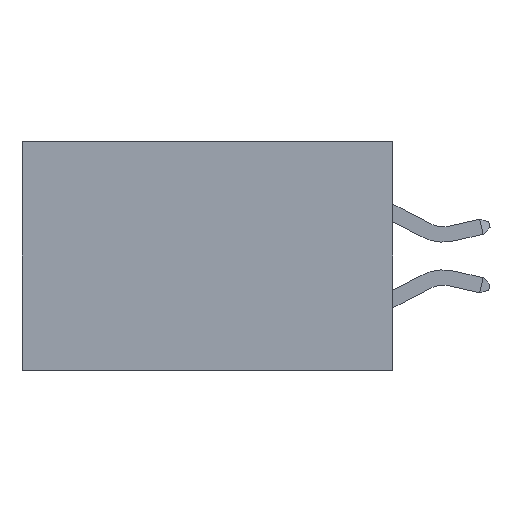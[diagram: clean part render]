
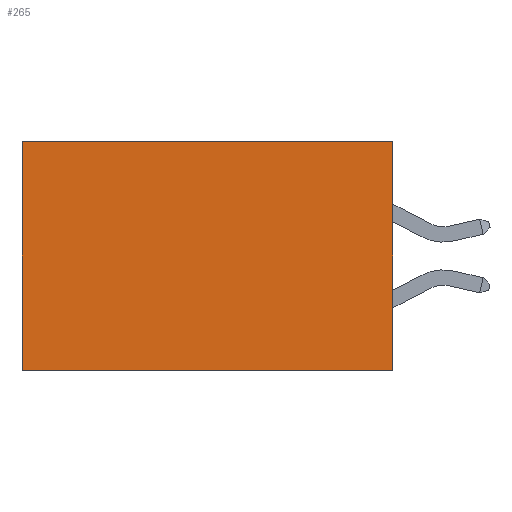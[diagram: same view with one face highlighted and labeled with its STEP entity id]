
A CAD part, left-side view. The second image highlights one B-rep face of the part: STEP entity #265.
In plain terms, the highlighted planar face has unit normal (-1, 0, 0).
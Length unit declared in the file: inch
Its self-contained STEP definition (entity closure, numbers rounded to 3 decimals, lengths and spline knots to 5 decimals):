
#207 = LINE ( 'NONE', #3480, #1048 ) ;
#265 = ADVANCED_FACE ( 'NONE', ( #1594 ), #11943, .F. ) ;
#588 = VERTEX_POINT ( 'NONE', #8306 ) ;
#1048 = VECTOR ( 'NONE', #12451, 39.37008 ) ;
#1594 = FACE_OUTER_BOUND ( 'NONE', #10352, .T. ) ;
#1827 = CARTESIAN_POINT ( 'NONE',  ( 0.2875, 0., -0.37 ) ) ;
#2550 = EDGE_CURVE ( 'NONE', #588, #6470, #16349, .T. ) ;
#2761 = DIRECTION ( 'NONE',  ( 0., 0., -1. ) ) ;
#3114 = CARTESIAN_POINT ( 'NONE',  ( 0.2875, 0., 0. ) ) ;
#3480 = CARTESIAN_POINT ( 'NONE',  ( 0.2875, 0.6, 0. ) ) ;
#3903 = LINE ( 'NONE', #1827, #13692 ) ;
#4053 = ORIENTED_EDGE ( 'NONE', *, *, #15684, .T. ) ;
#4161 = VECTOR ( 'NONE', #5811, 39.37008 ) ;
#4887 = CARTESIAN_POINT ( 'NONE',  ( 0.2875, 0., 0. ) ) ;
#5660 = DIRECTION ( 'NONE',  ( 1., 0., 0. ) ) ;
#5811 = DIRECTION ( 'NONE',  ( 0., 1., 0. ) ) ;
#6010 = VERTEX_POINT ( 'NONE', #13376 ) ;
#6470 = VERTEX_POINT ( 'NONE', #12179 ) ;
#6586 = EDGE_CURVE ( 'NONE', #6470, #6010, #3903, .T. ) ;
#6608 = VERTEX_POINT ( 'NONE', #8161 ) ;
#7960 = EDGE_CURVE ( 'NONE', #6608, #6010, #207, .T. ) ;
#8161 = CARTESIAN_POINT ( 'NONE',  ( 0.2875, 0.6, 0. ) ) ;
#8306 = CARTESIAN_POINT ( 'NONE',  ( 0.2875, 0., 0. ) ) ;
#10352 = EDGE_LOOP ( 'NONE', ( #15147, #13366, #12860, #4053 ) ) ;
#10518 = VECTOR ( 'NONE', #2761, 39.37008 ) ;
#10606 = AXIS2_PLACEMENT_3D ( 'NONE', #10685, #5660, #14445 ) ;
#10651 = DIRECTION ( 'NONE',  ( 0., 1., 0. ) ) ;
#10685 = CARTESIAN_POINT ( 'NONE',  ( 0.2875, 0., 0. ) ) ;
#11374 = LINE ( 'NONE', #3114, #4161 ) ;
#11943 = PLANE ( 'NONE',  #10606 ) ;
#12179 = CARTESIAN_POINT ( 'NONE',  ( 0.2875, 0., -0.37 ) ) ;
#12451 = DIRECTION ( 'NONE',  ( 0., 0., -1. ) ) ;
#12860 = ORIENTED_EDGE ( 'NONE', *, *, #2550, .F. ) ;
#13366 = ORIENTED_EDGE ( 'NONE', *, *, #6586, .F. ) ;
#13376 = CARTESIAN_POINT ( 'NONE',  ( 0.2875, 0.6, -0.37 ) ) ;
#13692 = VECTOR ( 'NONE', #10651, 39.37008 ) ;
#14445 = DIRECTION ( 'NONE',  ( 0., 0., -1. ) ) ;
#15147 = ORIENTED_EDGE ( 'NONE', *, *, #7960, .T. ) ;
#15684 = EDGE_CURVE ( 'NONE', #588, #6608, #11374, .T. ) ;
#16349 = LINE ( 'NONE', #4887, #10518 ) ;
